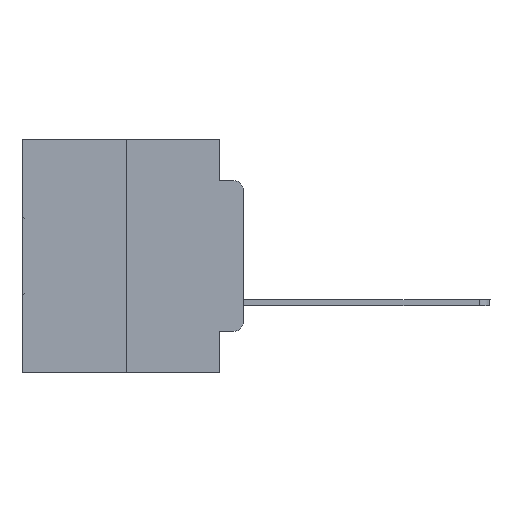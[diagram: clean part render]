
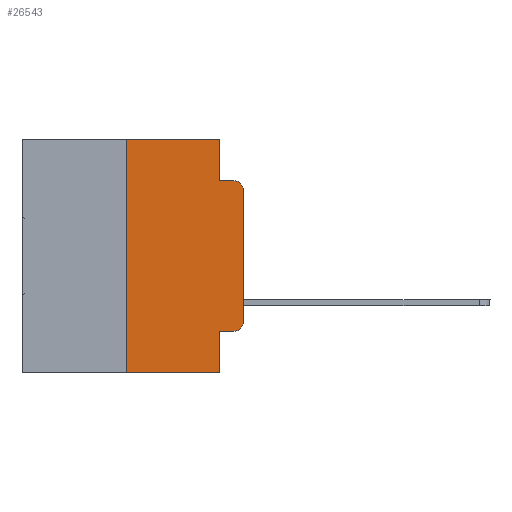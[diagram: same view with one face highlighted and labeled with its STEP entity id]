
A CAD part, left-side view. The second image highlights one B-rep face of the part: STEP entity #26543.
In plain terms, the highlighted planar face has unit normal (-1, 0, 0).
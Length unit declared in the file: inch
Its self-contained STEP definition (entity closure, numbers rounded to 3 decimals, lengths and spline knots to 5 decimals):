
#235 = ORIENTED_EDGE ( 'NONE', *, *, #12885, .T. ) ;
#557 = CARTESIAN_POINT ( 'NONE',  ( 0., 0.25, 0. ) ) ;
#810 = LINE ( 'NONE', #10843, #16287 ) ;
#873 = ORIENTED_EDGE ( 'NONE', *, *, #3513, .F. ) ;
#1084 = VECTOR ( 'NONE', #26520, 39.37008 ) ;
#1272 = DIRECTION ( 'NONE',  ( 0., -1., 0. ) ) ;
#1531 = CARTESIAN_POINT ( 'NONE',  ( 0., 0.051, -0.0885 ) ) ;
#2167 = DIRECTION ( 'NONE',  ( 0., 0., -1. ) ) ;
#2270 = PLANE ( 'NONE',  #23913 ) ;
#3264 = VERTEX_POINT ( 'NONE', #24855 ) ;
#3513 = EDGE_CURVE ( 'NONE', #9995, #15180, #30783, .T. ) ;
#3697 = CARTESIAN_POINT ( 'NONE',  ( 0., 0.02, -0.3915 ) ) ;
#3819 = ORIENTED_EDGE ( 'NONE', *, *, #7664, .F. ) ;
#4073 = VECTOR ( 'NONE', #27497, 39.37008 ) ;
#5207 = CARTESIAN_POINT ( 'NONE',  ( 0., 0., 0. ) ) ;
#5917 = CARTESIAN_POINT ( 'NONE',  ( 0., 0.02, -0.0885 ) ) ;
#6216 = VECTOR ( 'NONE', #17273, 39.37008 ) ;
#6824 = VECTOR ( 'NONE', #27884, 39.37008 ) ;
#7592 = CARTESIAN_POINT ( 'NONE',  ( 0., 0.02, -0.1085 ) ) ;
#7664 = EDGE_CURVE ( 'NONE', #15180, #8300, #23312, .T. ) ;
#8291 = VERTEX_POINT ( 'NONE', #21501 ) ;
#8300 = VERTEX_POINT ( 'NONE', #23525 ) ;
#9274 = CARTESIAN_POINT ( 'NONE',  ( 0., 0.473, 0. ) ) ;
#9624 = VECTOR ( 'NONE', #14098, 39.37008 ) ;
#9756 = LINE ( 'NONE', #5207, #21481 ) ;
#9904 = ORIENTED_EDGE ( 'NONE', *, *, #15724, .F. ) ;
#9995 = VERTEX_POINT ( 'NONE', #30998 ) ;
#10843 = CARTESIAN_POINT ( 'NONE',  ( 0., 0.051, -0.4115 ) ) ;
#11266 = DIRECTION ( 'NONE',  ( 0., 0., -1. ) ) ;
#11346 = EDGE_CURVE ( 'NONE', #3264, #8291, #19280, .T. ) ;
#11349 = EDGE_CURVE ( 'NONE', #14097, #3264, #810, .T. ) ;
#12425 = DIRECTION ( 'NONE',  ( -1., 0., 0. ) ) ;
#12885 = EDGE_CURVE ( 'NONE', #29963, #14541, #15401, .T. ) ;
#13156 = ORIENTED_EDGE ( 'NONE', *, *, #13696, .T. ) ;
#13696 = EDGE_CURVE ( 'NONE', #24774, #14981, #25605, .T. ) ;
#14097 = VERTEX_POINT ( 'NONE', #18103 ) ;
#14098 = DIRECTION ( 'NONE',  ( 0., -1., 0. ) ) ;
#14541 = VERTEX_POINT ( 'NONE', #5917 ) ;
#14808 = CARTESIAN_POINT ( 'NONE',  ( 0., 0.051, -0.5 ) ) ;
#14981 = VERTEX_POINT ( 'NONE', #14808 ) ;
#15114 = CARTESIAN_POINT ( 'NONE',  ( 0., 0.051, 0. ) ) ;
#15180 = VERTEX_POINT ( 'NONE', #15528 ) ;
#15401 = CIRCLE ( 'NONE', #15497, 0.02 ) ;
#15497 = AXIS2_PLACEMENT_3D ( 'NONE', #7592, #12425, #29130 ) ;
#15528 = CARTESIAN_POINT ( 'NONE',  ( 0., 0.051, 0. ) ) ;
#15724 = EDGE_CURVE ( 'NONE', #24774, #9995, #20924, .T. ) ;
#16240 = ORIENTED_EDGE ( 'NONE', *, *, #11346, .T. ) ;
#16287 = VECTOR ( 'NONE', #1272, 39.37008 ) ;
#17273 = DIRECTION ( 'NONE',  ( 0., 0., 1. ) ) ;
#18103 = CARTESIAN_POINT ( 'NONE',  ( 0., 0.051, -0.4115 ) ) ;
#18124 = VECTOR ( 'NONE', #21716, 39.37008 ) ;
#18439 = EDGE_CURVE ( 'NONE', #8300, #14541, #22656, .T. ) ;
#18639 = ORIENTED_EDGE ( 'NONE', *, *, #18439, .F. ) ;
#19280 = CIRCLE ( 'NONE', #26802, 0.02 ) ;
#19779 = EDGE_CURVE ( 'NONE', #14097, #14981, #24568, .T. ) ;
#20442 = CARTESIAN_POINT ( 'NONE',  ( 0., 0.051, 0. ) ) ;
#20924 = LINE ( 'NONE', #557, #6216 ) ;
#21082 = EDGE_CURVE ( 'NONE', #8291, #29963, #9756, .T. ) ;
#21481 = VECTOR ( 'NONE', #29635, 39.37008 ) ;
#21501 = CARTESIAN_POINT ( 'NONE',  ( 0., 0., -0.3915 ) ) ;
#21716 = DIRECTION ( 'NONE',  ( 0., 0., -1. ) ) ;
#22656 = LINE ( 'NONE', #1531, #6824 ) ;
#23171 = ORIENTED_EDGE ( 'NONE', *, *, #11349, .T. ) ;
#23312 = LINE ( 'NONE', #20442, #4073 ) ;
#23525 = CARTESIAN_POINT ( 'NONE',  ( 0., 0.051, -0.0885 ) ) ;
#23907 = EDGE_LOOP ( 'NONE', ( #25710, #235, #18639, #3819, #873, #9904, #13156, #24802, #23171, #16240 ) ) ;
#23913 = AXIS2_PLACEMENT_3D ( 'NONE', #31208, #28536, #2167 ) ;
#24073 = CARTESIAN_POINT ( 'NONE',  ( 0., 0.473, -0.5 ) ) ;
#24568 = LINE ( 'NONE', #15114, #18124 ) ;
#24774 = VERTEX_POINT ( 'NONE', #29661 ) ;
#24802 = ORIENTED_EDGE ( 'NONE', *, *, #19779, .F. ) ;
#24855 = CARTESIAN_POINT ( 'NONE',  ( 0., 0.02, -0.4115 ) ) ;
#25194 = FACE_OUTER_BOUND ( 'NONE', #23907, .T. ) ;
#25605 = LINE ( 'NONE', #24073, #1084 ) ;
#25710 = ORIENTED_EDGE ( 'NONE', *, *, #21082, .T. ) ;
#25715 = DIRECTION ( 'NONE',  ( -1., 0., 0. ) ) ;
#26520 = DIRECTION ( 'NONE',  ( 0., -1., 0. ) ) ;
#26543 = ADVANCED_FACE ( 'NONE', ( #25194 ), #2270, .F. ) ;
#26802 = AXIS2_PLACEMENT_3D ( 'NONE', #3697, #25715, #11266 ) ;
#27407 = CARTESIAN_POINT ( 'NONE',  ( 0., 0., -0.1085 ) ) ;
#27497 = DIRECTION ( 'NONE',  ( 0., 0., -1. ) ) ;
#27884 = DIRECTION ( 'NONE',  ( 0., -1., 0. ) ) ;
#28536 = DIRECTION ( 'NONE',  ( 1., 0., 0. ) ) ;
#29130 = DIRECTION ( 'NONE',  ( 0., 0., -1. ) ) ;
#29635 = DIRECTION ( 'NONE',  ( 0., 0., 1. ) ) ;
#29661 = CARTESIAN_POINT ( 'NONE',  ( 0., 0.25, -0.5 ) ) ;
#29963 = VERTEX_POINT ( 'NONE', #27407 ) ;
#30783 = LINE ( 'NONE', #9274, #9624 ) ;
#30998 = CARTESIAN_POINT ( 'NONE',  ( 0., 0.25, 0. ) ) ;
#31208 = CARTESIAN_POINT ( 'NONE',  ( 0., 0.473, 0. ) ) ;
